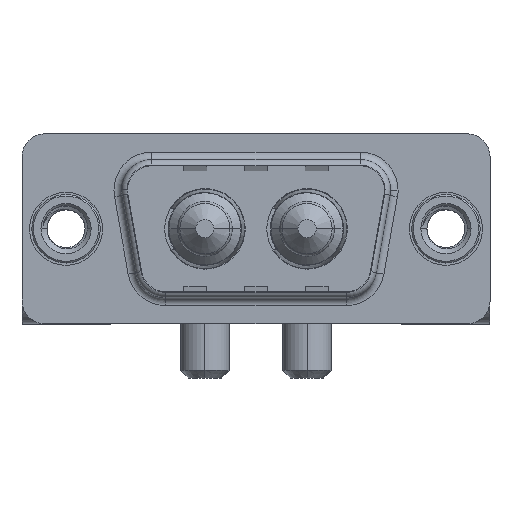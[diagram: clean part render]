
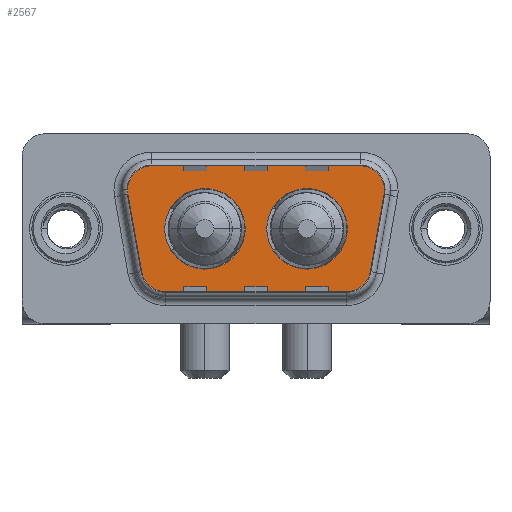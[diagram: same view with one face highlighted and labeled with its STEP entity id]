
A CAD part, top view. The second image highlights one B-rep face of the part: STEP entity #2567.
In plain terms, the highlighted planar face has unit normal (0, 0, 1).
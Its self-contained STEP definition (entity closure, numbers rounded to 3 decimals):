
#351 = EDGE_CURVE ( 'NONE', #13333, #9452, #9840, .T. ) ;
#392 = DIRECTION ( 'NONE',  ( -1., 0., 0. ) ) ;
#579 = LINE ( 'NONE', #11615, #13303 ) ;
#599 = VERTEX_POINT ( 'NONE', #6668 ) ;
#622 = EDGE_CURVE ( 'NONE', #599, #10250, #13288, .T. ) ;
#667 = CARTESIAN_POINT ( 'NONE',  ( 15.86, 0., 0. ) ) ;
#748 = DIRECTION ( 'NONE',  ( 1., 0., 0. ) ) ;
#932 = VECTOR ( 'NONE', #6846, 1000. ) ;
#1133 = CIRCLE ( 'NONE', #9103, 2.65 ) ;
#1243 = DIRECTION ( 'NONE',  ( 0., 0., 1. ) ) ;
#1424 = FACE_BOUND ( 'NONE', #5976, .T. ) ;
#1518 = VERTEX_POINT ( 'NONE', #5347 ) ;
#1591 = AXIS2_PLACEMENT_3D ( 'NONE', #4685, #7804, #392 ) ;
#1796 = VERTEX_POINT ( 'NONE', #10784 ) ;
#1810 = CARTESIAN_POINT ( 'NONE',  ( 18.541, -2.9, 0. ) ) ;
#1951 = CARTESIAN_POINT ( 'NONE',  ( 5.436, 2.9, 0. ) ) ;
#2017 = EDGE_CURVE ( 'NONE', #1518, #8007, #2143, .T. ) ;
#2030 = DIRECTION ( 'NONE',  ( 1., 0., 0. ) ) ;
#2096 = CARTESIAN_POINT ( 'NONE',  ( 9.14, 0., 0. ) ) ;
#2143 = LINE ( 'NONE', #6512, #12241 ) ;
#2237 = CARTESIAN_POINT ( 'NONE',  ( 18.541, -4.9, 0. ) ) ;
#2264 = VERTEX_POINT ( 'NONE', #12398 ) ;
#2411 = LINE ( 'NONE', #2703, #5017 ) ;
#2567 = ADVANCED_FACE ( 'NONE', ( #7978, #1424, #3709 ), #5706, .T. ) ;
#2625 = EDGE_CURVE ( 'NONE', #9452, #599, #2411, .T. ) ;
#2698 = VERTEX_POINT ( 'NONE', #10409 ) ;
#2703 = CARTESIAN_POINT ( 'NONE',  ( 21.534, 2.553, 0. ) ) ;
#2957 = DIRECTION ( 'NONE',  ( 1., 0., 0. ) ) ;
#3056 = ORIENTED_EDGE ( 'NONE', *, *, #2017, .T. ) ;
#3176 = DIRECTION ( 'NONE',  ( 1., 0., 0. ) ) ;
#3399 = CARTESIAN_POINT ( 'NONE',  ( 20.511, -3.247, 0. ) ) ;
#3415 = EDGE_CURVE ( 'NONE', #1796, #8917, #1133, .T. ) ;
#3480 = EDGE_CURVE ( 'NONE', #8917, #1796, #3875, .T. ) ;
#3576 = EDGE_CURVE ( 'NONE', #10250, #1518, #4099, .T. ) ;
#3695 = AXIS2_PLACEMENT_3D ( 'NONE', #1810, #8372, #2957 ) ;
#3709 = FACE_OUTER_BOUND ( 'NONE', #4146, .T. ) ;
#3740 = ORIENTED_EDGE ( 'NONE', *, *, #5138, .T. ) ;
#3823 = ORIENTED_EDGE ( 'NONE', *, *, #3576, .T. ) ;
#3859 = VERTEX_POINT ( 'NONE', #11030 ) ;
#3875 = CIRCLE ( 'NONE', #13645, 2.65 ) ;
#3904 = DIRECTION ( 'NONE',  ( 0., 0., 1. ) ) ;
#4006 = CIRCLE ( 'NONE', #4927, 2. ) ;
#4099 = CIRCLE ( 'NONE', #1591, 2. ) ;
#4144 = CARTESIAN_POINT ( 'NONE',  ( 6.459, -2.9, 0. ) ) ;
#4146 = EDGE_LOOP ( 'NONE', ( #8175, #8288, #10032, #3823, #3056, #8118, #10472, #6225, #3740 ) ) ;
#4182 = CARTESIAN_POINT ( 'NONE',  ( 9.14, 0., 0. ) ) ;
#4533 = DIRECTION ( 'NONE',  ( -1., 0., 0. ) ) ;
#4667 = CARTESIAN_POINT ( 'NONE',  ( 6.459, -4.9, 0. ) ) ;
#4685 = CARTESIAN_POINT ( 'NONE',  ( 19.564, 2.9, 0. ) ) ;
#4895 = AXIS2_PLACEMENT_3D ( 'NONE', #667, #4952, #6306 ) ;
#4927 = AXIS2_PLACEMENT_3D ( 'NONE', #4144, #13751, #8343 ) ;
#4952 = DIRECTION ( 'NONE',  ( 0., 0., 1. ) ) ;
#5017 = VECTOR ( 'NONE', #7062, 1000. ) ;
#5138 = EDGE_CURVE ( 'NONE', #11877, #13333, #9979, .T. ) ;
#5347 = CARTESIAN_POINT ( 'NONE',  ( 19.564, 4.9, 0. ) ) ;
#5706 = PLANE ( 'NONE',  #7721 ) ;
#5842 = DIRECTION ( 'NONE',  ( 1., 0., 0. ) ) ;
#5874 = AXIS2_PLACEMENT_3D ( 'NONE', #8111, #3904, #5842 ) ;
#5976 = EDGE_LOOP ( 'NONE', ( #12208, #14040 ) ) ;
#6015 = DIRECTION ( 'NONE',  ( 0.174, -0.985, 0. ) ) ;
#6017 = EDGE_LOOP ( 'NONE', ( #11147, #10771 ) ) ;
#6225 = ORIENTED_EDGE ( 'NONE', *, *, #12013, .T. ) ;
#6306 = DIRECTION ( 'NONE',  ( 1., 0., 0. ) ) ;
#6512 = CARTESIAN_POINT ( 'NONE',  ( 5.436, 4.9, 0. ) ) ;
#6552 = CIRCLE ( 'NONE', #5874, 2.65 ) ;
#6668 = CARTESIAN_POINT ( 'NONE',  ( 21.534, 2.553, 0. ) ) ;
#6846 = DIRECTION ( 'NONE',  ( 1., 0., 0. ) ) ;
#6988 = DIRECTION ( 'NONE',  ( 0., 0., 1. ) ) ;
#7062 = DIRECTION ( 'NONE',  ( 0.174, 0.985, 0. ) ) ;
#7161 = AXIS2_PLACEMENT_3D ( 'NONE', #7728, #1243, #4533 ) ;
#7621 = CIRCLE ( 'NONE', #4895, 2.65 ) ;
#7715 = DIRECTION ( 'NONE',  ( -1., 0., 0. ) ) ;
#7721 = AXIS2_PLACEMENT_3D ( 'NONE', #12314, #6988, #10050 ) ;
#7728 = CARTESIAN_POINT ( 'NONE',  ( 19.564, 2.9, 0. ) ) ;
#7772 = VERTEX_POINT ( 'NONE', #10620 ) ;
#7804 = DIRECTION ( 'NONE',  ( 0., 0., 1. ) ) ;
#7905 = CARTESIAN_POINT ( 'NONE',  ( 6.459, -4.9, 0. ) ) ;
#7978 = FACE_BOUND ( 'NONE', #6017, .T. ) ;
#8007 = VERTEX_POINT ( 'NONE', #8477 ) ;
#8096 = CARTESIAN_POINT ( 'NONE',  ( 11.79, 0., 0. ) ) ;
#8111 = CARTESIAN_POINT ( 'NONE',  ( 15.86, 0., 0. ) ) ;
#8118 = ORIENTED_EDGE ( 'NONE', *, *, #9800, .T. ) ;
#8175 = ORIENTED_EDGE ( 'NONE', *, *, #351, .T. ) ;
#8288 = ORIENTED_EDGE ( 'NONE', *, *, #2625, .T. ) ;
#8343 = DIRECTION ( 'NONE',  ( -1., 0., 0. ) ) ;
#8372 = DIRECTION ( 'NONE',  ( 0., 0., 1. ) ) ;
#8477 = CARTESIAN_POINT ( 'NONE',  ( 5.436, 4.9, 0. ) ) ;
#8741 = CIRCLE ( 'NONE', #9900, 2. ) ;
#8917 = VERTEX_POINT ( 'NONE', #8096 ) ;
#9103 = AXIS2_PLACEMENT_3D ( 'NONE', #4182, #11933, #3176 ) ;
#9452 = VERTEX_POINT ( 'NONE', #3399 ) ;
#9800 = EDGE_CURVE ( 'NONE', #8007, #7772, #8741, .T. ) ;
#9840 = CIRCLE ( 'NONE', #3695, 2. ) ;
#9900 = AXIS2_PLACEMENT_3D ( 'NONE', #1951, #10523, #748 ) ;
#9979 = LINE ( 'NONE', #7905, #932 ) ;
#10032 = ORIENTED_EDGE ( 'NONE', *, *, #622, .T. ) ;
#10050 = DIRECTION ( 'NONE',  ( 1., 0., 0. ) ) ;
#10250 = VERTEX_POINT ( 'NONE', #11430 ) ;
#10299 = EDGE_CURVE ( 'NONE', #3859, #2698, #7621, .T. ) ;
#10409 = CARTESIAN_POINT ( 'NONE',  ( 18.51, 0., 0. ) ) ;
#10472 = ORIENTED_EDGE ( 'NONE', *, *, #10712, .T. ) ;
#10523 = DIRECTION ( 'NONE',  ( 0., 0., 1. ) ) ;
#10620 = CARTESIAN_POINT ( 'NONE',  ( 3.466, 2.553, 0. ) ) ;
#10712 = EDGE_CURVE ( 'NONE', #7772, #2264, #579, .T. ) ;
#10771 = ORIENTED_EDGE ( 'NONE', *, *, #10299, .F. ) ;
#10784 = CARTESIAN_POINT ( 'NONE',  ( 6.49, 0., 0. ) ) ;
#11030 = CARTESIAN_POINT ( 'NONE',  ( 13.21, 0., 0. ) ) ;
#11147 = ORIENTED_EDGE ( 'NONE', *, *, #13514, .F. ) ;
#11430 = CARTESIAN_POINT ( 'NONE',  ( 21.564, 2.9, 0. ) ) ;
#11615 = CARTESIAN_POINT ( 'NONE',  ( 3.466, 2.553, 0. ) ) ;
#11877 = VERTEX_POINT ( 'NONE', #4667 ) ;
#11933 = DIRECTION ( 'NONE',  ( 0., 0., 1. ) ) ;
#12013 = EDGE_CURVE ( 'NONE', #2264, #11877, #4006, .T. ) ;
#12208 = ORIENTED_EDGE ( 'NONE', *, *, #3480, .F. ) ;
#12241 = VECTOR ( 'NONE', #7715, 1000. ) ;
#12314 = CARTESIAN_POINT ( 'NONE',  ( 18.541, -2.9, 0. ) ) ;
#12398 = CARTESIAN_POINT ( 'NONE',  ( 4.489, -3.247, 0. ) ) ;
#12856 = DIRECTION ( 'NONE',  ( 0., 0., 1. ) ) ;
#13288 = CIRCLE ( 'NONE', #7161, 2. ) ;
#13303 = VECTOR ( 'NONE', #6015, 1000. ) ;
#13333 = VERTEX_POINT ( 'NONE', #2237 ) ;
#13514 = EDGE_CURVE ( 'NONE', #2698, #3859, #6552, .T. ) ;
#13645 = AXIS2_PLACEMENT_3D ( 'NONE', #2096, #12856, #2030 ) ;
#13751 = DIRECTION ( 'NONE',  ( 0., 0., 1. ) ) ;
#14040 = ORIENTED_EDGE ( 'NONE', *, *, #3415, .F. ) ;
